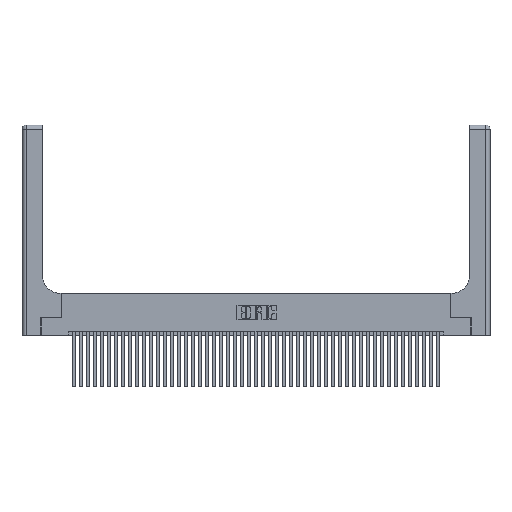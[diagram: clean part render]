
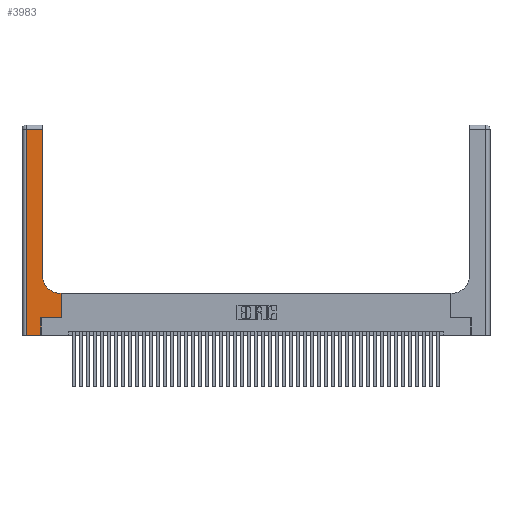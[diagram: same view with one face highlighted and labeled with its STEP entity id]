
A CAD part, top view. The second image highlights one B-rep face of the part: STEP entity #3983.
In plain terms, the highlighted planar face has unit normal (0, 0, 1).
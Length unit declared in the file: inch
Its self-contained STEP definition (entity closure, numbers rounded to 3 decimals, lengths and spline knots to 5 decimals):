
#62 = LINE ( 'NONE', #29207, #32734 ) ;
#510 = ORIENTED_EDGE ( 'NONE', *, *, #19179, .T. ) ;
#657 = VERTEX_POINT ( 'NONE', #9850 ) ;
#903 = CARTESIAN_POINT ( 'NONE',  ( 0.2915, 3., 0.37 ) ) ;
#1186 = VECTOR ( 'NONE', #20992, 39.37008 ) ;
#2391 = VECTOR ( 'NONE', #21693, 39.37008 ) ;
#3366 = EDGE_CURVE ( 'NONE', #657, #37198, #19663, .T. ) ;
#3791 = PLANE ( 'NONE',  #7683 ) ;
#3943 = DIRECTION ( 'NONE',  ( 0., 0., -1. ) ) ;
#3983 = ADVANCED_FACE ( 'NONE', ( #43674 ), #3791, .F. ) ;
#4170 = DIRECTION ( 'NONE',  ( 0., 0., -1. ) ) ;
#4235 = LINE ( 'NONE', #14467, #26079 ) ;
#4628 = CARTESIAN_POINT ( 'NONE',  ( 0.5415, 0.85, 0.37 ) ) ;
#4651 = EDGE_CURVE ( 'NONE', #8571, #21503, #4235, .T. ) ;
#5934 = EDGE_CURVE ( 'NONE', #23445, #20698, #20476, .T. ) ;
#7014 = ORIENTED_EDGE ( 'NONE', *, *, #5934, .T. ) ;
#7683 = AXIS2_PLACEMENT_3D ( 'NONE', #31699, #3943, #25101 ) ;
#7922 = DIRECTION ( 'NONE',  ( 0., 1., 0. ) ) ;
#8571 = VERTEX_POINT ( 'NONE', #21669 ) ;
#9850 = CARTESIAN_POINT ( 'NONE',  ( 0.06, 0., 0.37 ) ) ;
#10137 = CARTESIAN_POINT ( 'NONE',  ( 0.2915, 0.85, 0.37 ) ) ;
#10794 = CARTESIAN_POINT ( 'NONE',  ( 0., 2.94, 0.37 ) ) ;
#10996 = CARTESIAN_POINT ( 'NONE',  ( 0.5585, 0.25, 0.37 ) ) ;
#12682 = LINE ( 'NONE', #10794, #1186 ) ;
#14467 = CARTESIAN_POINT ( 'NONE',  ( 0.2915, 0.6, 0.37 ) ) ;
#15321 = DIRECTION ( 'NONE',  ( 1., 0., 0. ) ) ;
#18739 = VERTEX_POINT ( 'NONE', #35349 ) ;
#19161 = CARTESIAN_POINT ( 'NONE',  ( 0.5415, 0.6, 0.37 ) ) ;
#19179 = EDGE_CURVE ( 'NONE', #20698, #28241, #12682, .T. ) ;
#19663 = LINE ( 'NONE', #38691, #44821 ) ;
#19977 = EDGE_CURVE ( 'NONE', #18739, #35401, #62, .T. ) ;
#20476 = LINE ( 'NONE', #903, #34174 ) ;
#20698 = VERTEX_POINT ( 'NONE', #23751 ) ;
#20992 = DIRECTION ( 'NONE',  ( -1., 0., 0. ) ) ;
#21314 = LINE ( 'NONE', #29126, #30111 ) ;
#21503 = VERTEX_POINT ( 'NONE', #19161 ) ;
#21669 = CARTESIAN_POINT ( 'NONE',  ( 0.5585, 0.6, 0.37 ) ) ;
#21693 = DIRECTION ( 'NONE',  ( 0., -1., 0. ) ) ;
#21912 = ORIENTED_EDGE ( 'NONE', *, *, #40532, .T. ) ;
#21984 = CARTESIAN_POINT ( 'NONE',  ( 0.06, 2.94, 0.37 ) ) ;
#23445 = VERTEX_POINT ( 'NONE', #10137 ) ;
#23751 = CARTESIAN_POINT ( 'NONE',  ( 0.2915, 2.94, 0.37 ) ) ;
#25101 = DIRECTION ( 'NONE',  ( -1., 0., 0. ) ) ;
#25169 = DIRECTION ( 'NONE',  ( 1., 0., 0. ) ) ;
#26079 = VECTOR ( 'NONE', #42731, 39.37008 ) ;
#28241 = VERTEX_POINT ( 'NONE', #21984 ) ;
#28505 = EDGE_CURVE ( 'NONE', #28241, #657, #34555, .T. ) ;
#29020 = CIRCLE ( 'NONE', #39323, 0.25 ) ;
#29126 = CARTESIAN_POINT ( 'NONE',  ( 0.269, 0., 0.37 ) ) ;
#29207 = CARTESIAN_POINT ( 'NONE',  ( 0.269, 0.25, 0.37 ) ) ;
#30010 = ORIENTED_EDGE ( 'NONE', *, *, #28505, .T. ) ;
#30111 = VECTOR ( 'NONE', #35993, 39.37008 ) ;
#30541 = LINE ( 'NONE', #33306, #42003 ) ;
#30700 = EDGE_LOOP ( 'NONE', ( #7014, #510, #30010, #41048, #21912, #30750, #38016, #38302, #44206 ) ) ;
#30750 = ORIENTED_EDGE ( 'NONE', *, *, #19977, .T. ) ;
#31699 = CARTESIAN_POINT ( 'NONE',  ( 0., 3., 0.37 ) ) ;
#32734 = VECTOR ( 'NONE', #15321, 39.37008 ) ;
#33156 = DIRECTION ( 'NONE',  ( 0., 1., 0. ) ) ;
#33306 = CARTESIAN_POINT ( 'NONE',  ( 0.5585, 0.25, 0.37 ) ) ;
#34174 = VECTOR ( 'NONE', #7922, 39.37008 ) ;
#34555 = LINE ( 'NONE', #35330, #2391 ) ;
#35034 = EDGE_CURVE ( 'NONE', #21503, #23445, #29020, .T. ) ;
#35330 = CARTESIAN_POINT ( 'NONE',  ( 0.06, 3., 0.37 ) ) ;
#35349 = CARTESIAN_POINT ( 'NONE',  ( 0.269, 0.25, 0.37 ) ) ;
#35401 = VERTEX_POINT ( 'NONE', #10996 ) ;
#35639 = DIRECTION ( 'NONE',  ( 1., 0., 0. ) ) ;
#35993 = DIRECTION ( 'NONE',  ( 0., 1., 0. ) ) ;
#37198 = VERTEX_POINT ( 'NONE', #43948 ) ;
#38016 = ORIENTED_EDGE ( 'NONE', *, *, #41577, .T. ) ;
#38302 = ORIENTED_EDGE ( 'NONE', *, *, #4651, .T. ) ;
#38691 = CARTESIAN_POINT ( 'NONE',  ( 0., 0., 0.37 ) ) ;
#39323 = AXIS2_PLACEMENT_3D ( 'NONE', #4628, #4170, #25169 ) ;
#40532 = EDGE_CURVE ( 'NONE', #37198, #18739, #21314, .T. ) ;
#41048 = ORIENTED_EDGE ( 'NONE', *, *, #3366, .T. ) ;
#41577 = EDGE_CURVE ( 'NONE', #35401, #8571, #30541, .T. ) ;
#42003 = VECTOR ( 'NONE', #33156, 39.37008 ) ;
#42731 = DIRECTION ( 'NONE',  ( -1., 0., 0. ) ) ;
#43674 = FACE_OUTER_BOUND ( 'NONE', #30700, .T. ) ;
#43948 = CARTESIAN_POINT ( 'NONE',  ( 0.269, 0., 0.37 ) ) ;
#44206 = ORIENTED_EDGE ( 'NONE', *, *, #35034, .T. ) ;
#44821 = VECTOR ( 'NONE', #35639, 39.37008 ) ;
